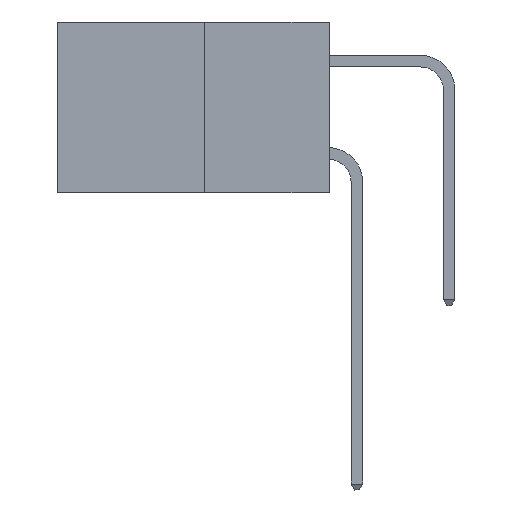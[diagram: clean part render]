
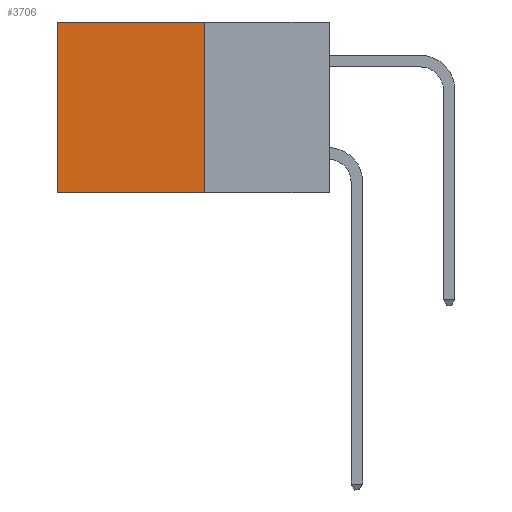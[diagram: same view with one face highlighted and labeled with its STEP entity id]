
A CAD part, left-side view. The second image highlights one B-rep face of the part: STEP entity #3706.
In plain terms, the highlighted planar face has unit normal (-1, 0, 0).
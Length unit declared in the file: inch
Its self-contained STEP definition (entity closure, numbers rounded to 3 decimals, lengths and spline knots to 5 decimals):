
#1444 = VECTOR ( 'NONE', #10706, 39.37008 ) ;
#1449 = ORIENTED_EDGE ( 'NONE', *, *, #2355, .F. ) ;
#1928 = LINE ( 'NONE', #10843, #1444 ) ;
#2321 = PLANE ( 'NONE',  #2832 ) ;
#2355 = EDGE_CURVE ( 'NONE', #9567, #6519, #8853, .T. ) ;
#2549 = VECTOR ( 'NONE', #3894, 39.37008 ) ;
#2832 = AXIS2_PLACEMENT_3D ( 'NONE', #19284, #5782, #15466 ) ;
#3100 = EDGE_CURVE ( 'NONE', #12877, #6519, #18928, .T. ) ;
#3706 = ADVANCED_FACE ( 'NONE', ( #16557 ), #2321, .F. ) ;
#3811 = CARTESIAN_POINT ( 'NONE',  ( 0.277, 0.27, 0. ) ) ;
#3894 = DIRECTION ( 'NONE',  ( 0., 0., -1. ) ) ;
#4354 = CARTESIAN_POINT ( 'NONE',  ( 0.277, 0.59, -0.37 ) ) ;
#4555 = ORIENTED_EDGE ( 'NONE', *, *, #11903, .F. ) ;
#5782 = DIRECTION ( 'NONE',  ( 1., 0., 0. ) ) ;
#6519 = VERTEX_POINT ( 'NONE', #6909 ) ;
#6786 = VERTEX_POINT ( 'NONE', #3811 ) ;
#6909 = CARTESIAN_POINT ( 'NONE',  ( 0.277, 0.59, -0.37 ) ) ;
#7350 = LINE ( 'NONE', #9848, #15092 ) ;
#8385 = VECTOR ( 'NONE', #14793, 39.37008 ) ;
#8853 = LINE ( 'NONE', #13662, #8385 ) ;
#9567 = VERTEX_POINT ( 'NONE', #12903 ) ;
#9682 = DIRECTION ( 'NONE',  ( 0., 0., -1. ) ) ;
#9834 = EDGE_CURVE ( 'NONE', #6786, #12877, #1928, .T. ) ;
#9848 = CARTESIAN_POINT ( 'NONE',  ( 0.277, 0.27, -0.37 ) ) ;
#10368 = ORIENTED_EDGE ( 'NONE', *, *, #3100, .T. ) ;
#10706 = DIRECTION ( 'NONE',  ( 0., 1., 0. ) ) ;
#10843 = CARTESIAN_POINT ( 'NONE',  ( 0.277, 0.27, 0. ) ) ;
#11903 = EDGE_CURVE ( 'NONE', #6786, #9567, #7350, .T. ) ;
#12877 = VERTEX_POINT ( 'NONE', #14456 ) ;
#12903 = CARTESIAN_POINT ( 'NONE',  ( 0.277, 0.27, -0.37 ) ) ;
#13662 = CARTESIAN_POINT ( 'NONE',  ( 0.277, 0.27, -0.37 ) ) ;
#14456 = CARTESIAN_POINT ( 'NONE',  ( 0.277, 0.59, 0. ) ) ;
#14793 = DIRECTION ( 'NONE',  ( 0., 1., 0. ) ) ;
#15092 = VECTOR ( 'NONE', #9682, 39.37008 ) ;
#15466 = DIRECTION ( 'NONE',  ( 0., 0., -1. ) ) ;
#16377 = EDGE_LOOP ( 'NONE', ( #10368, #1449, #4555, #17817 ) ) ;
#16557 = FACE_OUTER_BOUND ( 'NONE', #16377, .T. ) ;
#17817 = ORIENTED_EDGE ( 'NONE', *, *, #9834, .T. ) ;
#18928 = LINE ( 'NONE', #4354, #2549 ) ;
#19284 = CARTESIAN_POINT ( 'NONE',  ( 0.277, 0.27, -0.37 ) ) ;
